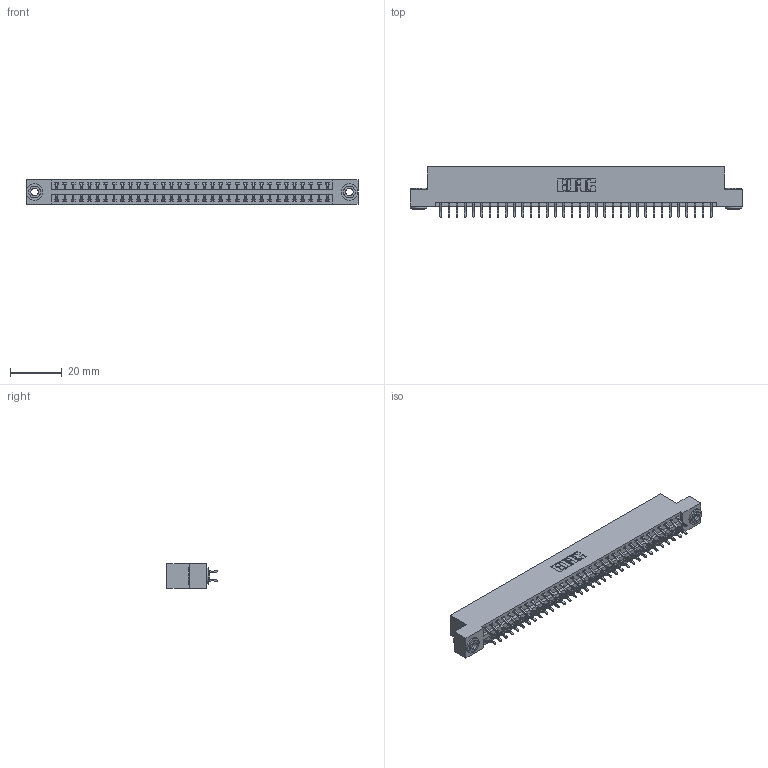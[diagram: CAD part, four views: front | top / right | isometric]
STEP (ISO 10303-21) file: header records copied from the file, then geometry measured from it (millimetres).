
FILE_DESCRIPTION (( 'STEP AP203' ), '1' );
FILE_NAME ('346-068-556-203.STEP', '2022-05-24T19:48:41', ( '' ), ( '' ), 'SwSTEP 2.0', 'SolidWorks 2020', '' );
FILE_SCHEMA (( 'CONFIG_CONTROL_DESIGN' ));
Length unit declared in the file: inch
Products named in the file (4): 345-292-001_556 Tail; 345-250-002_345-250-002-102; 346 Part_Flush Mounting Lugs - 0.156 Dia-TH; 346-068-556-203
Assembly tree (71 placements, depth 2):
  346-068-556-203
    346 Part_Flush Mounting Lugs - 0.156 Dia-TH
    345-292-001_556 Tail  x68
    345-250-002_345-250-002-102  x2
Bounding box: 128.52 x 19.57 x 9.4 mm (x, y, z)
Volume: 12469.2 mm3; surface area: 17199.5 mm2
Topology: 71 solids, 71 shells, 4118 faces, 12205 edges, 8042 vertices
Faces by surface type: plane 2752, cylinder 1358, cone 8
Entity records: 24552 total; most frequent: CARTESIAN_POINT 4053, ORIENTED_EDGE 3966, DIRECTION 3641, EDGE_CURVE 1983, LINE 1683, VECTOR 1683, VERTEX_POINT 1318, AXIS2_PLACEMENT_3D 979
